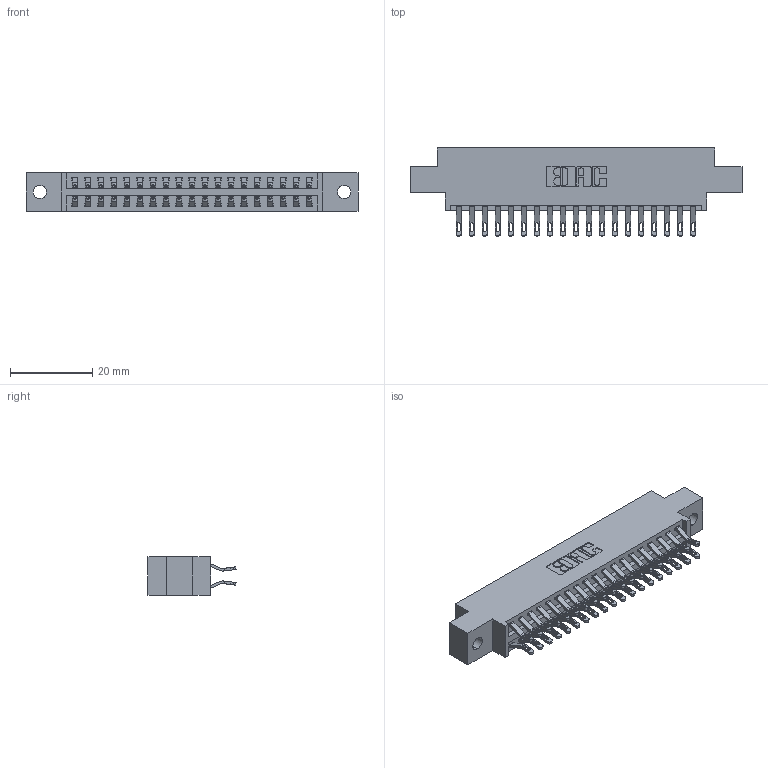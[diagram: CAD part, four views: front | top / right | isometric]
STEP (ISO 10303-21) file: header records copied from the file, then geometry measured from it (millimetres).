
FILE_DESCRIPTION (( 'STEP AP203' ), '1' );
FILE_NAME ('346-038-555-802.STEP', '2022-05-20T00:06:54', ( '' ), ( '' ), 'SwSTEP 2.0', 'SolidWorks 2020', '' );
FILE_SCHEMA (( 'CONFIG_CONTROL_DESIGN' ));
Length unit declared in the file: inch
Products named in the file (3): 345-292-001_555 Tail; 346-038-555-802; 346 Part_0.170 Offset - 0.128 Dia
Assembly tree (39 placements, depth 2):
  346-038-555-802
    346 Part_0.170 Offset - 0.128 Dia
    345-292-001_555 Tail  x38
Bounding box: 80.9 x 21.46 x 9.4 mm (x, y, z)
Volume: 7628.9 mm3; surface area: 10428.3 mm2
Topology: 39 solids, 39 shells, 2330 faces, 7295 edges, 4862 vertices
Faces by surface type: plane 1334, cylinder 996
Entity records: 15957 total; most frequent: CARTESIAN_POINT 2698, ORIENTED_EDGE 2602, DIRECTION 2397, EDGE_CURVE 1301, VECTOR 1073, LINE 1073, VERTEX_POINT 866, AXIS2_PLACEMENT_3D 662
